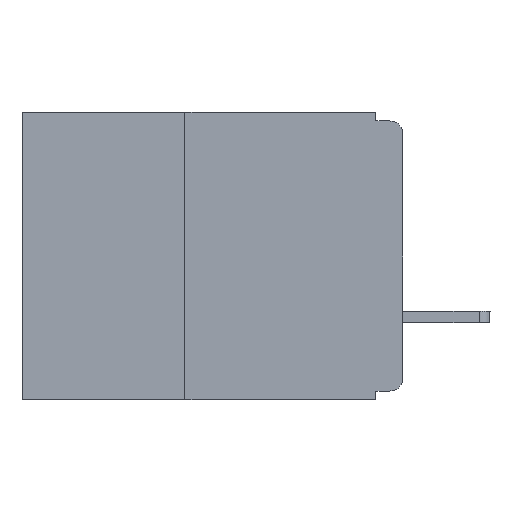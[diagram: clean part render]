
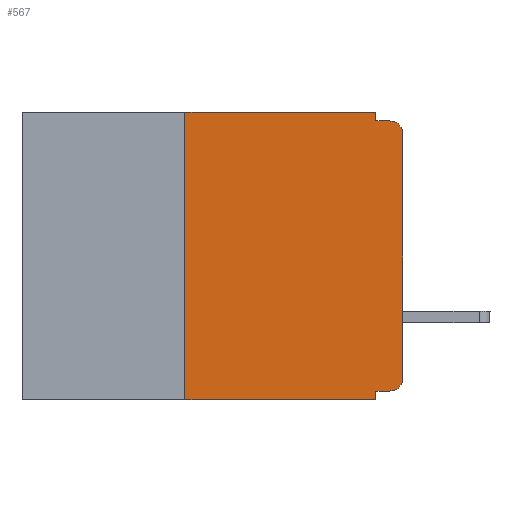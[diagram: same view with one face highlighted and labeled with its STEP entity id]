
A CAD part, left-side view. The second image highlights one B-rep face of the part: STEP entity #567.
In plain terms, the highlighted planar face has unit normal (-1, 0, 0).
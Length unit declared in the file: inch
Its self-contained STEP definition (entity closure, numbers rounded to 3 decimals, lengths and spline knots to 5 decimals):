
#74 = CARTESIAN_POINT ( 'NONE',  ( 0., 0.015, -0.025 ) ) ;
#87 = ORIENTED_EDGE ( 'NONE', *, *, #1911, .T. ) ;
#174 = CIRCLE ( 'NONE', #1568, 0.015 ) ;
#210 = VERTEX_POINT ( 'NONE', #7407 ) ;
#511 = VECTOR ( 'NONE', #8832, 39.37008 ) ;
#567 = ADVANCED_FACE ( 'NONE', ( #2200 ), #6956, .F. ) ;
#571 = LINE ( 'NONE', #10694, #8201 ) ;
#634 = CARTESIAN_POINT ( 'NONE',  ( 0., 0.031, -0.01 ) ) ;
#914 = ORIENTED_EDGE ( 'NONE', *, *, #4491, .F. ) ;
#1259 = CARTESIAN_POINT ( 'NONE',  ( 0., 0.25, -0.33 ) ) ;
#1568 = AXIS2_PLACEMENT_3D ( 'NONE', #74, #7085, #7040 ) ;
#1742 = CARTESIAN_POINT ( 'NONE',  ( 0., 0., -0.025 ) ) ;
#1911 = EDGE_CURVE ( 'NONE', #210, #1914, #571, .T. ) ;
#1914 = VERTEX_POINT ( 'NONE', #1742 ) ;
#1958 = DIRECTION ( 'NONE',  ( 0., 0., 1. ) ) ;
#2200 = FACE_OUTER_BOUND ( 'NONE', #6979, .T. ) ;
#2603 = VECTOR ( 'NONE', #5772, 39.37008 ) ;
#2686 = ORIENTED_EDGE ( 'NONE', *, *, #8544, .T. ) ;
#2700 = CARTESIAN_POINT ( 'NONE',  ( 0., 0., -0.01 ) ) ;
#2734 = LINE ( 'NONE', #6105, #6446 ) ;
#3214 = ORIENTED_EDGE ( 'NONE', *, *, #9836, .F. ) ;
#3483 = VECTOR ( 'NONE', #8537, 39.37008 ) ;
#3699 = CARTESIAN_POINT ( 'NONE',  ( 0., 0.015, -0.305 ) ) ;
#3810 = CARTESIAN_POINT ( 'NONE',  ( 0., 0.015, -0.01 ) ) ;
#3827 = LINE ( 'NONE', #4687, #2603 ) ;
#4206 = EDGE_CURVE ( 'NONE', #11975, #6746, #6291, .T. ) ;
#4491 = EDGE_CURVE ( 'NONE', #6746, #4568, #4900, .T. ) ;
#4519 = EDGE_CURVE ( 'NONE', #11300, #6790, #5502, .T. ) ;
#4568 = VERTEX_POINT ( 'NONE', #3810 ) ;
#4647 = EDGE_CURVE ( 'NONE', #10216, #6790, #12207, .T. ) ;
#4683 = CARTESIAN_POINT ( 'NONE',  ( 0., 0.437, -0.33 ) ) ;
#4687 = CARTESIAN_POINT ( 'NONE',  ( 0., 0.437, 0. ) ) ;
#4775 = CARTESIAN_POINT ( 'NONE',  ( 0., 0.031, -0.32 ) ) ;
#4900 = LINE ( 'NONE', #2700, #9998 ) ;
#4981 = AXIS2_PLACEMENT_3D ( 'NONE', #3699, #10655, #11682 ) ;
#5195 = DIRECTION ( 'NONE',  ( 0., 1., 0. ) ) ;
#5294 = ORIENTED_EDGE ( 'NONE', *, *, #9022, .F. ) ;
#5502 = LINE ( 'NONE', #4683, #3483 ) ;
#5565 = CARTESIAN_POINT ( 'NONE',  ( 0., 0.031, -0.33 ) ) ;
#5772 = DIRECTION ( 'NONE',  ( 0., -1., 0. ) ) ;
#6071 = AXIS2_PLACEMENT_3D ( 'NONE', #11089, #6132, #9062 ) ;
#6105 = CARTESIAN_POINT ( 'NONE',  ( 0., 0., -0.32 ) ) ;
#6132 = DIRECTION ( 'NONE',  ( 1., 0., 0. ) ) ;
#6291 = LINE ( 'NONE', #11933, #12505 ) ;
#6446 = VECTOR ( 'NONE', #5195, 39.37008 ) ;
#6734 = DIRECTION ( 'NONE',  ( 0., 0., 1. ) ) ;
#6746 = VERTEX_POINT ( 'NONE', #634 ) ;
#6790 = VERTEX_POINT ( 'NONE', #5565 ) ;
#6941 = CIRCLE ( 'NONE', #4981, 0.015 ) ;
#6956 = PLANE ( 'NONE',  #6071 ) ;
#6979 = EDGE_LOOP ( 'NONE', ( #87, #7890, #914, #8927, #5294, #3214, #8115, #8899, #7501, #2686 ) ) ;
#7040 = DIRECTION ( 'NONE',  ( 0., 0., -1. ) ) ;
#7085 = DIRECTION ( 'NONE',  ( -1., 0., 0. ) ) ;
#7407 = CARTESIAN_POINT ( 'NONE',  ( 0., 0., -0.305 ) ) ;
#7501 = ORIENTED_EDGE ( 'NONE', *, *, #12356, .F. ) ;
#7688 = VECTOR ( 'NONE', #1958, 39.37008 ) ;
#7728 = CARTESIAN_POINT ( 'NONE',  ( 0., 0.25, -0.33 ) ) ;
#7757 = VERTEX_POINT ( 'NONE', #9517 ) ;
#7852 = CARTESIAN_POINT ( 'NONE',  ( 0., 0.031, -0.33 ) ) ;
#7890 = ORIENTED_EDGE ( 'NONE', *, *, #11702, .T. ) ;
#7950 = DIRECTION ( 'NONE',  ( 0., 0., -1. ) ) ;
#8115 = ORIENTED_EDGE ( 'NONE', *, *, #4519, .T. ) ;
#8201 = VECTOR ( 'NONE', #6734, 39.37008 ) ;
#8537 = DIRECTION ( 'NONE',  ( 0., -1., 0. ) ) ;
#8544 = EDGE_CURVE ( 'NONE', #7757, #210, #6941, .T. ) ;
#8832 = DIRECTION ( 'NONE',  ( 0., 0., -1. ) ) ;
#8899 = ORIENTED_EDGE ( 'NONE', *, *, #4647, .F. ) ;
#8927 = ORIENTED_EDGE ( 'NONE', *, *, #4206, .F. ) ;
#9022 = EDGE_CURVE ( 'NONE', #12027, #11975, #3827, .T. ) ;
#9062 = DIRECTION ( 'NONE',  ( 0., 0., -1. ) ) ;
#9517 = CARTESIAN_POINT ( 'NONE',  ( 0., 0.015, -0.32 ) ) ;
#9836 = EDGE_CURVE ( 'NONE', #11300, #12027, #10314, .T. ) ;
#9998 = VECTOR ( 'NONE', #12496, 39.37008 ) ;
#10056 = CARTESIAN_POINT ( 'NONE',  ( 0., 0.031, 0. ) ) ;
#10216 = VERTEX_POINT ( 'NONE', #4775 ) ;
#10314 = LINE ( 'NONE', #7728, #7688 ) ;
#10655 = DIRECTION ( 'NONE',  ( -1., 0., 0. ) ) ;
#10694 = CARTESIAN_POINT ( 'NONE',  ( 0., 0., 0. ) ) ;
#11089 = CARTESIAN_POINT ( 'NONE',  ( 0., 0.437, 0. ) ) ;
#11300 = VERTEX_POINT ( 'NONE', #1259 ) ;
#11682 = DIRECTION ( 'NONE',  ( 0., 0., -1. ) ) ;
#11702 = EDGE_CURVE ( 'NONE', #1914, #4568, #174, .T. ) ;
#11933 = CARTESIAN_POINT ( 'NONE',  ( 0., 0.031, 0. ) ) ;
#11975 = VERTEX_POINT ( 'NONE', #10056 ) ;
#12027 = VERTEX_POINT ( 'NONE', #12094 ) ;
#12094 = CARTESIAN_POINT ( 'NONE',  ( 0., 0.25, 0. ) ) ;
#12207 = LINE ( 'NONE', #7852, #511 ) ;
#12356 = EDGE_CURVE ( 'NONE', #7757, #10216, #2734, .T. ) ;
#12496 = DIRECTION ( 'NONE',  ( 0., -1., 0. ) ) ;
#12505 = VECTOR ( 'NONE', #7950, 39.37008 ) ;
